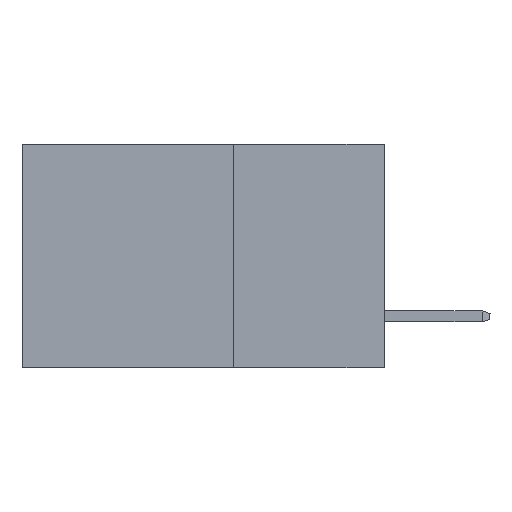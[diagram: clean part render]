
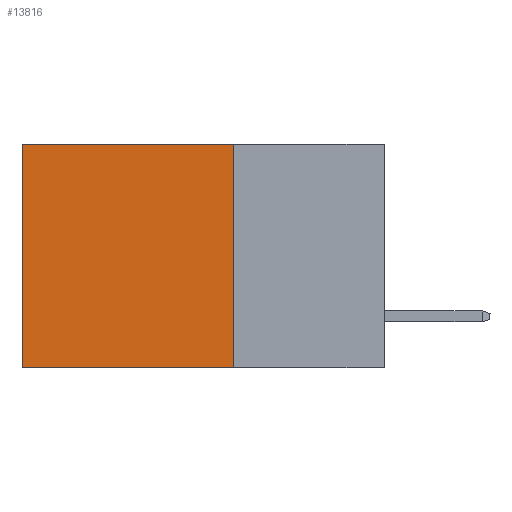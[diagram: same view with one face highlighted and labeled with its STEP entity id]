
A CAD part, left-side view. The second image highlights one B-rep face of the part: STEP entity #13816.
In plain terms, the highlighted planar face has unit normal (-1, 0, 0).
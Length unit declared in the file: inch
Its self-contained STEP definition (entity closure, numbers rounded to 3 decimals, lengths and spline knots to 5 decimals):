
#513 = CARTESIAN_POINT ( 'NONE',  ( 0.2615, 0.25, -0.37 ) ) ;
#1075 = VECTOR ( 'NONE', #10073, 39.37008 ) ;
#1396 = EDGE_LOOP ( 'NONE', ( #17368, #11734, #2538, #21494 ) ) ;
#2016 = DIRECTION ( 'NONE',  ( 0., 0., -1. ) ) ;
#2538 = ORIENTED_EDGE ( 'NONE', *, *, #14931, .F. ) ;
#3431 = FACE_OUTER_BOUND ( 'NONE', #1396, .T. ) ;
#4105 = VECTOR ( 'NONE', #19862, 39.37008 ) ;
#4645 = VERTEX_POINT ( 'NONE', #22728 ) ;
#5462 = VECTOR ( 'NONE', #5651, 39.37008 ) ;
#5651 = DIRECTION ( 'NONE',  ( 0., 1., 0. ) ) ;
#6051 = CARTESIAN_POINT ( 'NONE',  ( 0.2615, 0.25, 0. ) ) ;
#6828 = VERTEX_POINT ( 'NONE', #12273 ) ;
#7062 = EDGE_CURVE ( 'NONE', #10631, #4645, #19896, .T. ) ;
#7471 = EDGE_CURVE ( 'NONE', #8880, #6828, #9179, .T. ) ;
#8880 = VERTEX_POINT ( 'NONE', #6051 ) ;
#9179 = LINE ( 'NONE', #12910, #9381 ) ;
#9349 = AXIS2_PLACEMENT_3D ( 'NONE', #19466, #16166, #2016 ) ;
#9381 = VECTOR ( 'NONE', #16333, 39.37008 ) ;
#10073 = DIRECTION ( 'NONE',  ( 0., 0., -1. ) ) ;
#10631 = VERTEX_POINT ( 'NONE', #11339 ) ;
#11325 = CARTESIAN_POINT ( 'NONE',  ( 0.2615, 0.25, -0.37 ) ) ;
#11339 = CARTESIAN_POINT ( 'NONE',  ( 0.2615, 0.25, -0.37 ) ) ;
#11728 = LINE ( 'NONE', #17118, #1075 ) ;
#11734 = ORIENTED_EDGE ( 'NONE', *, *, #7062, .F. ) ;
#12273 = CARTESIAN_POINT ( 'NONE',  ( 0.2615, 0.6, 0. ) ) ;
#12289 = PLANE ( 'NONE',  #9349 ) ;
#12910 = CARTESIAN_POINT ( 'NONE',  ( 0.2615, 0.25, 0. ) ) ;
#13816 = ADVANCED_FACE ( 'NONE', ( #3431 ), #12289, .F. ) ;
#14931 = EDGE_CURVE ( 'NONE', #8880, #10631, #16680, .T. ) ;
#16166 = DIRECTION ( 'NONE',  ( 1., 0., 0. ) ) ;
#16333 = DIRECTION ( 'NONE',  ( 0., 1., 0. ) ) ;
#16616 = EDGE_CURVE ( 'NONE', #6828, #4645, #11728, .T. ) ;
#16680 = LINE ( 'NONE', #513, #4105 ) ;
#17118 = CARTESIAN_POINT ( 'NONE',  ( 0.2615, 0.6, -0.37 ) ) ;
#17368 = ORIENTED_EDGE ( 'NONE', *, *, #16616, .T. ) ;
#19466 = CARTESIAN_POINT ( 'NONE',  ( 0.2615, 0.25, -0.37 ) ) ;
#19862 = DIRECTION ( 'NONE',  ( 0., 0., -1. ) ) ;
#19896 = LINE ( 'NONE', #11325, #5462 ) ;
#21494 = ORIENTED_EDGE ( 'NONE', *, *, #7471, .T. ) ;
#22728 = CARTESIAN_POINT ( 'NONE',  ( 0.2615, 0.6, -0.37 ) ) ;
